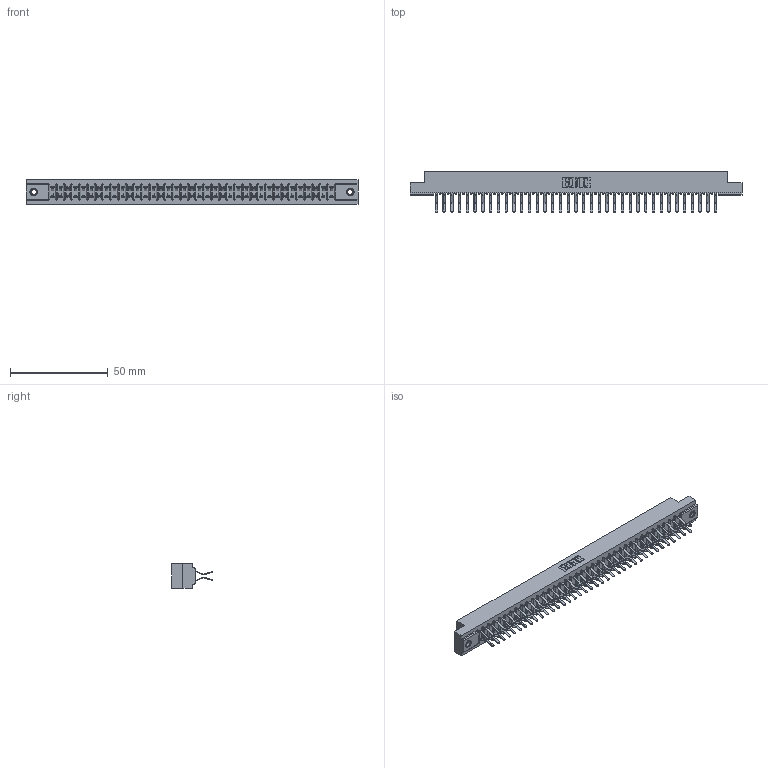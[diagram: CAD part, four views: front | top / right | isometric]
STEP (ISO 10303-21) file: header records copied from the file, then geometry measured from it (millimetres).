
FILE_DESCRIPTION (( 'STEP AP203' ), '1' );
FILE_NAME ('307-074-460-207.STEP', '2020-10-01T04:21:53', ( '' ), ( '' ), 'SwSTEP 2.0', 'SolidWorks 2020', '' );
FILE_SCHEMA (( 'CONFIG_CONTROL_DESIGN' ));
Length unit declared in the file: inch
Products named in the file (4): 307-290-001_560; 307 Part_.156 Dia Mounting Holes; 307-074-460-207; 345-250-001_345-250-005-103
Assembly tree (77 placements, depth 2):
  307-074-460-207
    307 Part_.156 Dia Mounting Holes
    307-290-001_560  x74
    345-250-001_345-250-005-103  x2
Bounding box: 169.62 x 20.73 x 12.7 mm (x, y, z)
Volume: 18080.5 mm3; surface area: 22551.5 mm2
Topology: 77 solids, 77 shells, 3916 faces, 10967 edges, 7102 vertices
Faces by surface type: plane 2544, cylinder 1280, sphere 76, cone 12, torus 4
Entity records: 34809 total; most frequent: CARTESIAN_POINT 5680, ORIENTED_EDGE 5622, DIRECTION 5575, EDGE_CURVE 2811, VECTOR 2153, LINE 2153, VERTEX_POINT 1816, AXIS2_PLACEMENT_3D 1711
